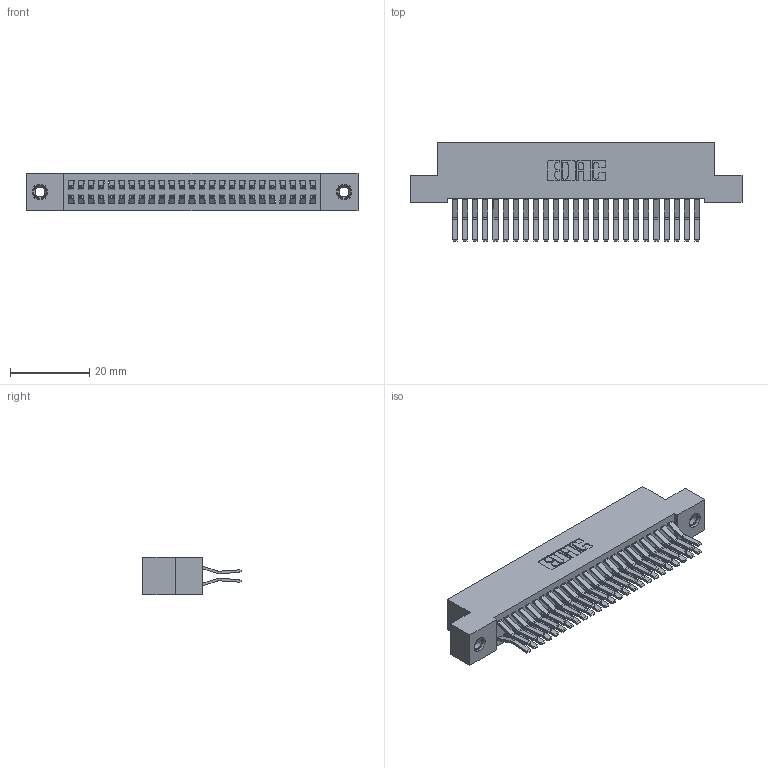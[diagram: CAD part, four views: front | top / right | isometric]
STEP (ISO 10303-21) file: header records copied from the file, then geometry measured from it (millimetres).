
FILE_DESCRIPTION (( 'STEP AP203' ), '1' );
FILE_NAME ('342-050-560-207.STEP', '2018-08-12T20:35:08', ( '' ), ( '' ), 'SwSTEP 2.0', 'SolidWorks 2016', '' );
FILE_SCHEMA (( 'CONFIG_CONTROL_DESIGN' ));
Length unit declared in the file: inch
Products named in the file (4): 345-292-001_560 Tail; 345-250-001_345-250-005-103; 342-050-560-207; 342 Part_TI
Assembly tree (53 placements, depth 2):
  342-050-560-207
    342 Part_TI
    345-292-001_560 Tail  x50
    345-250-001_345-250-005-103  x2
Bounding box: 83.82 x 24.78 x 9.4 mm (x, y, z)
Volume: 7766.3 mm3; surface area: 13035.7 mm2
Topology: 53 solids, 53 shells, 2870 faces, 8485 edges, 5582 vertices
Faces by surface type: plane 1898, cylinder 956, cone 12, torus 4
Entity records: 19424 total; most frequent: CARTESIAN_POINT 3221, ORIENTED_EDGE 3150, DIRECTION 2817, EDGE_CURVE 1575, VECTOR 1423, LINE 1423, VERTEX_POINT 1044, AXIS2_PLACEMENT_3D 697
